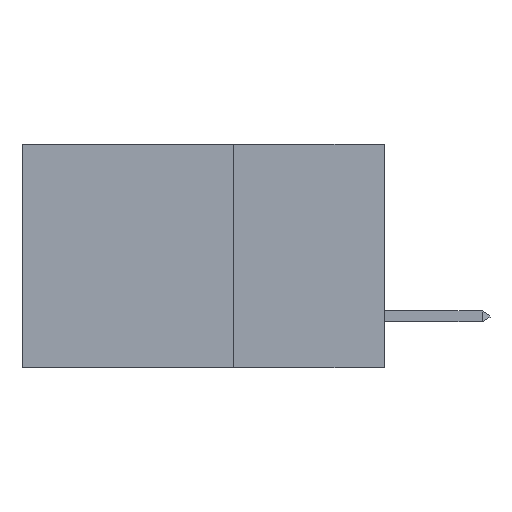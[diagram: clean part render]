
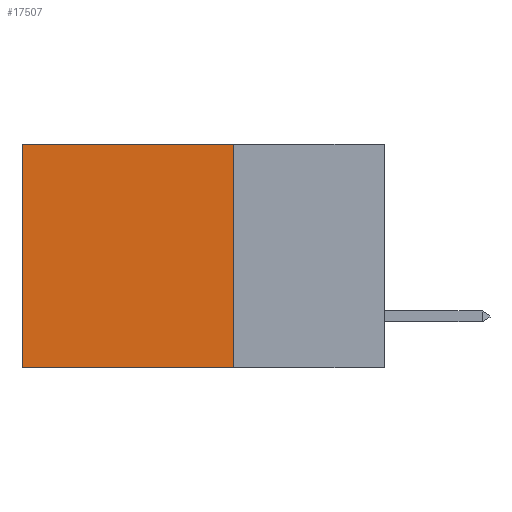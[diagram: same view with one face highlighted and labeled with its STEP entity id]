
A CAD part, left-side view. The second image highlights one B-rep face of the part: STEP entity #17507.
In plain terms, the highlighted planar face has unit normal (-1, 0, 0).
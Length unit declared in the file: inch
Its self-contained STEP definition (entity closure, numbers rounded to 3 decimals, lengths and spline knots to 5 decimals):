
#12 = DIRECTION ( 'NONE',  ( 0., 0., -1. ) ) ;
#45 = CARTESIAN_POINT ( 'NONE',  ( 0.2875, 0.25, 0. ) ) ;
#57 = CARTESIAN_POINT ( 'NONE',  ( 0.2875, 0.6, 0. ) ) ;
#619 = VERTEX_POINT ( 'NONE', #57 ) ;
#647 = CARTESIAN_POINT ( 'NONE',  ( 0.2875, 0.25, -0.37 ) ) ;
#865 = ORIENTED_EDGE ( 'NONE', *, *, #13516, .F. ) ;
#1327 = LINE ( 'NONE', #10920, #14273 ) ;
#3739 = CARTESIAN_POINT ( 'NONE',  ( 0.2875, 0.6, -0.37 ) ) ;
#3762 = DIRECTION ( 'NONE',  ( 0., 1., 0. ) ) ;
#4249 = CARTESIAN_POINT ( 'NONE',  ( 0.2875, 0.25, 0. ) ) ;
#5054 = ORIENTED_EDGE ( 'NONE', *, *, #11684, .T. ) ;
#5525 = CARTESIAN_POINT ( 'NONE',  ( 0.2875, 0.25, 0. ) ) ;
#6234 = VERTEX_POINT ( 'NONE', #3739 ) ;
#6311 = VECTOR ( 'NONE', #13107, 39.37008 ) ;
#6816 = DIRECTION ( 'NONE',  ( 0., 1., 0. ) ) ;
#7421 = LINE ( 'NONE', #17172, #6311 ) ;
#8214 = LINE ( 'NONE', #45, #12133 ) ;
#9510 = EDGE_CURVE ( 'NONE', #619, #6234, #7421, .T. ) ;
#9678 = DIRECTION ( 'NONE',  ( 1., 0., 0. ) ) ;
#9907 = CARTESIAN_POINT ( 'NONE',  ( 0.2875, 0.25, 0. ) ) ;
#10364 = ORIENTED_EDGE ( 'NONE', *, *, #14968, .F. ) ;
#10623 = EDGE_LOOP ( 'NONE', ( #10741, #865, #10364, #5054 ) ) ;
#10741 = ORIENTED_EDGE ( 'NONE', *, *, #9510, .T. ) ;
#10920 = CARTESIAN_POINT ( 'NONE',  ( 0.2875, 0.25, -0.37 ) ) ;
#11524 = DIRECTION ( 'NONE',  ( 0., 0., -1. ) ) ;
#11684 = EDGE_CURVE ( 'NONE', #13679, #619, #8214, .T. ) ;
#12133 = VECTOR ( 'NONE', #3762, 39.37008 ) ;
#12202 = AXIS2_PLACEMENT_3D ( 'NONE', #9907, #9678, #12 ) ;
#12767 = VECTOR ( 'NONE', #11524, 39.37008 ) ;
#13107 = DIRECTION ( 'NONE',  ( 0., 0., -1. ) ) ;
#13516 = EDGE_CURVE ( 'NONE', #15118, #6234, #1327, .T. ) ;
#13679 = VERTEX_POINT ( 'NONE', #5525 ) ;
#14273 = VECTOR ( 'NONE', #6816, 39.37008 ) ;
#14648 = FACE_OUTER_BOUND ( 'NONE', #10623, .T. ) ;
#14968 = EDGE_CURVE ( 'NONE', #13679, #15118, #16502, .T. ) ;
#15118 = VERTEX_POINT ( 'NONE', #647 ) ;
#16502 = LINE ( 'NONE', #4249, #12767 ) ;
#17172 = CARTESIAN_POINT ( 'NONE',  ( 0.2875, 0.6, 0. ) ) ;
#17507 = ADVANCED_FACE ( 'NONE', ( #14648 ), #18024, .F. ) ;
#18024 = PLANE ( 'NONE',  #12202 ) ;
